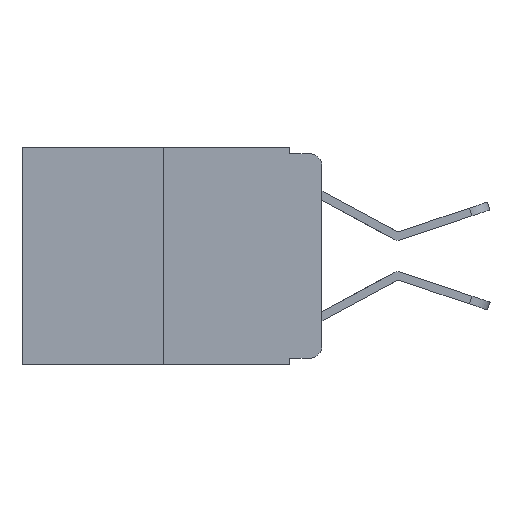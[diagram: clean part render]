
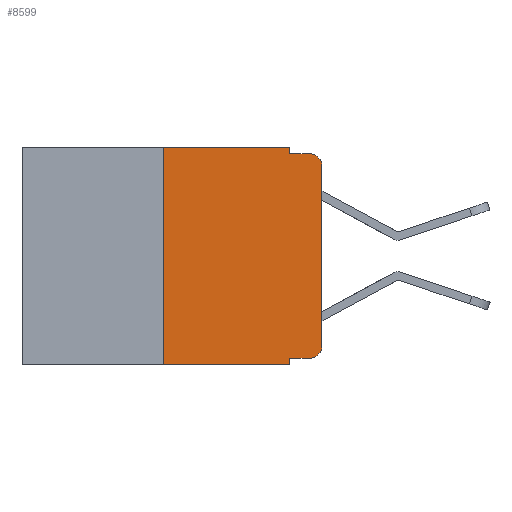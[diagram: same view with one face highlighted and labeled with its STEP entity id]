
A CAD part, left-side view. The second image highlights one B-rep face of the part: STEP entity #8599.
In plain terms, the highlighted planar face has unit normal (-1, 0, 0).
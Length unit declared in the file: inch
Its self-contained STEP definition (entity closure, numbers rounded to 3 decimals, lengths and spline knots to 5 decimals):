
#49 = CARTESIAN_POINT ( 'NONE',  ( 0., 0.051, -0.01 ) ) ;
#62 = ORIENTED_EDGE ( 'NONE', *, *, #271, .T. ) ;
#271 = EDGE_CURVE ( 'NONE', #10315, #7944, #3173, .T. ) ;
#381 = CARTESIAN_POINT ( 'NONE',  ( 0., 0.473, -0.343 ) ) ;
#436 = AXIS2_PLACEMENT_3D ( 'NONE', #3175, #3998, #5009 ) ;
#456 = CARTESIAN_POINT ( 'NONE',  ( 0., 0.25, -0.343 ) ) ;
#745 = ORIENTED_EDGE ( 'NONE', *, *, #1623, .F. ) ;
#805 = LINE ( 'NONE', #977, #6500 ) ;
#869 = CARTESIAN_POINT ( 'NONE',  ( 0., 0.02, -0.333 ) ) ;
#887 = EDGE_CURVE ( 'NONE', #8041, #10412, #10191, .T. ) ;
#968 = ORIENTED_EDGE ( 'NONE', *, *, #3870, .F. ) ;
#977 = CARTESIAN_POINT ( 'NONE',  ( 0., 0.051, -0.333 ) ) ;
#1036 = DIRECTION ( 'NONE',  ( 0., 0., -1. ) ) ;
#1114 = VECTOR ( 'NONE', #3046, 39.37008 ) ;
#1238 = EDGE_CURVE ( 'NONE', #10682, #2808, #6862, .T. ) ;
#1294 = DIRECTION ( 'NONE',  ( 0., -1., 0. ) ) ;
#1427 = ORIENTED_EDGE ( 'NONE', *, *, #4427, .T. ) ;
#1623 = EDGE_CURVE ( 'NONE', #10339, #10412, #11729, .T. ) ;
#1782 = LINE ( 'NONE', #11242, #9091 ) ;
#2365 = EDGE_CURVE ( 'NONE', #2808, #4065, #8127, .T. ) ;
#2653 = ORIENTED_EDGE ( 'NONE', *, *, #887, .T. ) ;
#2808 = VERTEX_POINT ( 'NONE', #10898 ) ;
#3023 = DIRECTION ( 'NONE',  ( 0., 0., -1. ) ) ;
#3046 = DIRECTION ( 'NONE',  ( 0., 0., 1. ) ) ;
#3115 = ORIENTED_EDGE ( 'NONE', *, *, #2365, .F. ) ;
#3155 = DIRECTION ( 'NONE',  ( 0., 0., -1. ) ) ;
#3173 = CIRCLE ( 'NONE', #436, 0.02 ) ;
#3175 = CARTESIAN_POINT ( 'NONE',  ( 0., 0.02, -0.313 ) ) ;
#3369 = VECTOR ( 'NONE', #1294, 39.37008 ) ;
#3666 = CARTESIAN_POINT ( 'NONE',  ( 0., 0.051, 0. ) ) ;
#3748 = EDGE_CURVE ( 'NONE', #9751, #4065, #3950, .T. ) ;
#3774 = CARTESIAN_POINT ( 'NONE',  ( 0., 0.25, 0. ) ) ;
#3870 = EDGE_CURVE ( 'NONE', #5178, #10682, #5807, .T. ) ;
#3950 = CIRCLE ( 'NONE', #8926, 0.02 ) ;
#3998 = DIRECTION ( 'NONE',  ( -1., 0., 0. ) ) ;
#4065 = VERTEX_POINT ( 'NONE', #6880 ) ;
#4427 = EDGE_CURVE ( 'NONE', #10339, #10315, #805, .T. ) ;
#4662 = CARTESIAN_POINT ( 'NONE',  ( 0., 0.473, 0. ) ) ;
#4769 = EDGE_CURVE ( 'NONE', #7944, #9751, #1782, .T. ) ;
#4923 = CARTESIAN_POINT ( 'NONE',  ( 0., 0.25, 0. ) ) ;
#5009 = DIRECTION ( 'NONE',  ( 0., 0., -1. ) ) ;
#5070 = CARTESIAN_POINT ( 'NONE',  ( 0., 0.473, 0. ) ) ;
#5075 = CARTESIAN_POINT ( 'NONE',  ( 0., 0.051, -0.333 ) ) ;
#5178 = VERTEX_POINT ( 'NONE', #3774 ) ;
#5489 = DIRECTION ( 'NONE',  ( -1., 0., 0. ) ) ;
#5734 = EDGE_LOOP ( 'NONE', ( #6462, #9227, #3115, #7678, #968, #10990, #2653, #745, #1427, #62 ) ) ;
#5789 = FACE_OUTER_BOUND ( 'NONE', #5734, .T. ) ;
#5807 = LINE ( 'NONE', #4662, #3369 ) ;
#6223 = CARTESIAN_POINT ( 'NONE',  ( 0., 0.051, -0.343 ) ) ;
#6286 = CARTESIAN_POINT ( 'NONE',  ( 0., 0.02, -0.03 ) ) ;
#6385 = LINE ( 'NONE', #4923, #1114 ) ;
#6462 = ORIENTED_EDGE ( 'NONE', *, *, #4769, .T. ) ;
#6500 = VECTOR ( 'NONE', #9364, 39.37008 ) ;
#6862 = LINE ( 'NONE', #11229, #9879 ) ;
#6880 = CARTESIAN_POINT ( 'NONE',  ( 0., 0.02, -0.01 ) ) ;
#7433 = EDGE_CURVE ( 'NONE', #8041, #5178, #6385, .T. ) ;
#7678 = ORIENTED_EDGE ( 'NONE', *, *, #1238, .F. ) ;
#7944 = VERTEX_POINT ( 'NONE', #9308 ) ;
#8013 = CARTESIAN_POINT ( 'NONE',  ( 0., 0.051, 0. ) ) ;
#8041 = VERTEX_POINT ( 'NONE', #456 ) ;
#8127 = LINE ( 'NONE', #49, #11146 ) ;
#8179 = DIRECTION ( 'NONE',  ( 0., 0., -1. ) ) ;
#8454 = DIRECTION ( 'NONE',  ( 0., 0., 1. ) ) ;
#8599 = ADVANCED_FACE ( 'NONE', ( #5789 ), #10431, .F. ) ;
#8926 = AXIS2_PLACEMENT_3D ( 'NONE', #6286, #5489, #8179 ) ;
#9091 = VECTOR ( 'NONE', #8454, 39.37008 ) ;
#9227 = ORIENTED_EDGE ( 'NONE', *, *, #3748, .T. ) ;
#9284 = CARTESIAN_POINT ( 'NONE',  ( 0., 0., -0.03 ) ) ;
#9308 = CARTESIAN_POINT ( 'NONE',  ( 0., 0., -0.313 ) ) ;
#9364 = DIRECTION ( 'NONE',  ( 0., -1., 0. ) ) ;
#9604 = DIRECTION ( 'NONE',  ( 1., 0., 0. ) ) ;
#9610 = VECTOR ( 'NONE', #10401, 39.37008 ) ;
#9722 = VECTOR ( 'NONE', #1036, 39.37008 ) ;
#9751 = VERTEX_POINT ( 'NONE', #9284 ) ;
#9879 = VECTOR ( 'NONE', #3023, 39.37008 ) ;
#10039 = DIRECTION ( 'NONE',  ( 0., -1., 0. ) ) ;
#10191 = LINE ( 'NONE', #381, #9610 ) ;
#10315 = VERTEX_POINT ( 'NONE', #869 ) ;
#10339 = VERTEX_POINT ( 'NONE', #5075 ) ;
#10401 = DIRECTION ( 'NONE',  ( 0., -1., 0. ) ) ;
#10412 = VERTEX_POINT ( 'NONE', #6223 ) ;
#10431 = PLANE ( 'NONE',  #11407 ) ;
#10682 = VERTEX_POINT ( 'NONE', #8013 ) ;
#10898 = CARTESIAN_POINT ( 'NONE',  ( 0., 0.051, -0.01 ) ) ;
#10990 = ORIENTED_EDGE ( 'NONE', *, *, #7433, .F. ) ;
#11146 = VECTOR ( 'NONE', #10039, 39.37008 ) ;
#11229 = CARTESIAN_POINT ( 'NONE',  ( 0., 0.051, 0. ) ) ;
#11242 = CARTESIAN_POINT ( 'NONE',  ( 0., 0., 0. ) ) ;
#11407 = AXIS2_PLACEMENT_3D ( 'NONE', #5070, #9604, #3155 ) ;
#11729 = LINE ( 'NONE', #3666, #9722 ) ;
